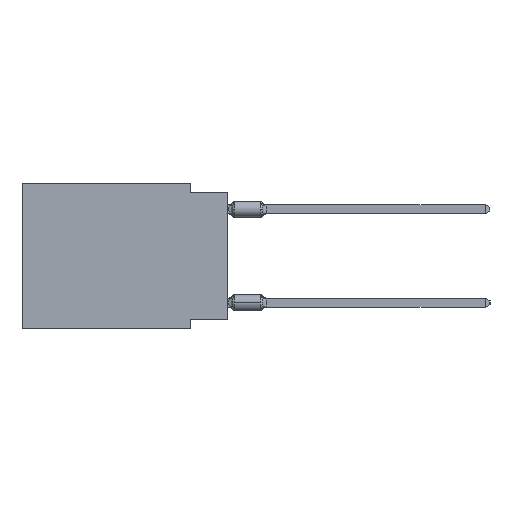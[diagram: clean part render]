
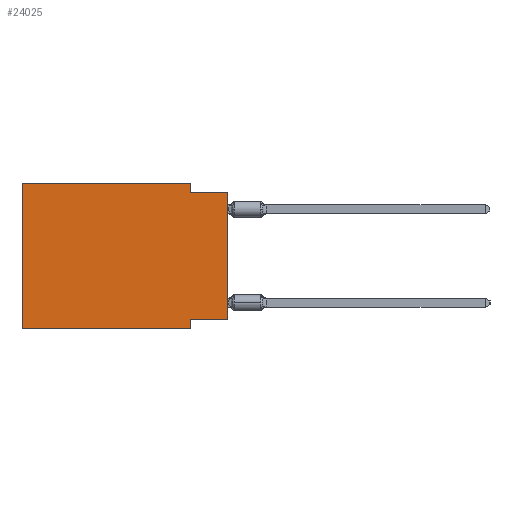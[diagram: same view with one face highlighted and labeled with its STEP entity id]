
A CAD part, left-side view. The second image highlights one B-rep face of the part: STEP entity #24025.
In plain terms, the highlighted planar face has unit normal (-1, 0, 0).
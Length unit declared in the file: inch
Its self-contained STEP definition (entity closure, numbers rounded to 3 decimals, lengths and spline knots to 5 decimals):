
#186 = DIRECTION ( 'NONE',  ( 0., 0., -1. ) ) ;
#632 = LINE ( 'NONE', #25896, #49363 ) ;
#1411 = EDGE_CURVE ( 'NONE', #21787, #33160, #45205, .T. ) ;
#2446 = LINE ( 'NONE', #11648, #55852 ) ;
#2876 = DIRECTION ( 'NONE',  ( 0., -1., 0. ) ) ;
#4531 = EDGE_CURVE ( 'NONE', #33160, #37035, #17638, .T. ) ;
#4639 = VERTEX_POINT ( 'NONE', #9086 ) ;
#4641 = LINE ( 'NONE', #53505, #16126 ) ;
#7725 = VECTOR ( 'NONE', #46171, 39.37008 ) ;
#8576 = VECTOR ( 'NONE', #23397, 39.37008 ) ;
#9086 = CARTESIAN_POINT ( 'NONE',  ( 0., 0.55, -0.39 ) ) ;
#10463 = EDGE_CURVE ( 'NONE', #4639, #32710, #58477, .T. ) ;
#11090 = CARTESIAN_POINT ( 'NONE',  ( 0., 0.1, 0. ) ) ;
#11648 = CARTESIAN_POINT ( 'NONE',  ( 0., 0.55, 0. ) ) ;
#12163 = EDGE_CURVE ( 'NONE', #59722, #14822, #4641, .T. ) ;
#12637 = EDGE_LOOP ( 'NONE', ( #64023, #55850, #13127, #46720, #32402, #53237, #25804, #24884 ) ) ;
#12735 = CARTESIAN_POINT ( 'NONE',  ( 0., 0., -0.025 ) ) ;
#13127 = ORIENTED_EDGE ( 'NONE', *, *, #1411, .F. ) ;
#14822 = VERTEX_POINT ( 'NONE', #28301 ) ;
#16050 = DIRECTION ( 'NONE',  ( 0., -1., 0. ) ) ;
#16126 = VECTOR ( 'NONE', #24639, 39.37008 ) ;
#16457 = CARTESIAN_POINT ( 'NONE',  ( 0., 0.1, -0.025 ) ) ;
#17084 = CARTESIAN_POINT ( 'NONE',  ( 0., 0.1, -0.39 ) ) ;
#17638 = LINE ( 'NONE', #12735, #24336 ) ;
#20513 = PLANE ( 'NONE',  #43126 ) ;
#21787 = VERTEX_POINT ( 'NONE', #56785 ) ;
#23397 = DIRECTION ( 'NONE',  ( 0., 0., 1. ) ) ;
#24025 = ADVANCED_FACE ( 'NONE', ( #35272 ), #20513, .F. ) ;
#24336 = VECTOR ( 'NONE', #2876, 39.37008 ) ;
#24639 = DIRECTION ( 'NONE',  ( 0., 1., 0. ) ) ;
#24884 = ORIENTED_EDGE ( 'NONE', *, *, #12163, .F. ) ;
#25804 = ORIENTED_EDGE ( 'NONE', *, *, #47475, .F. ) ;
#25896 = CARTESIAN_POINT ( 'NONE',  ( 0., 0.55, -0.39 ) ) ;
#27677 = EDGE_CURVE ( 'NONE', #32710, #21787, #2446, .T. ) ;
#28301 = CARTESIAN_POINT ( 'NONE',  ( 0., 0.1, -0.365 ) ) ;
#29759 = VECTOR ( 'NONE', #56361, 39.37008 ) ;
#32402 = ORIENTED_EDGE ( 'NONE', *, *, #10463, .F. ) ;
#32710 = VERTEX_POINT ( 'NONE', #53068 ) ;
#32928 = VECTOR ( 'NONE', #47964, 39.37008 ) ;
#33160 = VERTEX_POINT ( 'NONE', #16457 ) ;
#35272 = FACE_OUTER_BOUND ( 'NONE', #12637, .T. ) ;
#35713 = CARTESIAN_POINT ( 'NONE',  ( 0., 0.1, -0.39 ) ) ;
#37035 = VERTEX_POINT ( 'NONE', #61209 ) ;
#41490 = DIRECTION ( 'NONE',  ( 0., -1., 0. ) ) ;
#42134 = EDGE_CURVE ( 'NONE', #4639, #54829, #632, .T. ) ;
#43126 = AXIS2_PLACEMENT_3D ( 'NONE', #45112, #62066, #186 ) ;
#45112 = CARTESIAN_POINT ( 'NONE',  ( 0., 0.55, 0. ) ) ;
#45205 = LINE ( 'NONE', #11090, #7725 ) ;
#45882 = LINE ( 'NONE', #35713, #29759 ) ;
#46171 = DIRECTION ( 'NONE',  ( 0., 0., -1. ) ) ;
#46720 = ORIENTED_EDGE ( 'NONE', *, *, #27677, .F. ) ;
#47475 = EDGE_CURVE ( 'NONE', #14822, #54829, #45882, .T. ) ;
#47944 = EDGE_CURVE ( 'NONE', #59722, #37035, #48612, .T. ) ;
#47964 = DIRECTION ( 'NONE',  ( 0., 0., 1. ) ) ;
#48612 = LINE ( 'NONE', #48935, #32928 ) ;
#48935 = CARTESIAN_POINT ( 'NONE',  ( 0., 0., 0. ) ) ;
#49293 = CARTESIAN_POINT ( 'NONE',  ( 0., 0.55, 0. ) ) ;
#49363 = VECTOR ( 'NONE', #16050, 39.37008 ) ;
#53068 = CARTESIAN_POINT ( 'NONE',  ( 0., 0.55, 0. ) ) ;
#53237 = ORIENTED_EDGE ( 'NONE', *, *, #42134, .T. ) ;
#53505 = CARTESIAN_POINT ( 'NONE',  ( 0., 0., -0.365 ) ) ;
#54829 = VERTEX_POINT ( 'NONE', #17084 ) ;
#55850 = ORIENTED_EDGE ( 'NONE', *, *, #4531, .F. ) ;
#55852 = VECTOR ( 'NONE', #41490, 39.37008 ) ;
#56361 = DIRECTION ( 'NONE',  ( 0., 0., -1. ) ) ;
#56785 = CARTESIAN_POINT ( 'NONE',  ( 0., 0.1, 0. ) ) ;
#58477 = LINE ( 'NONE', #49293, #8576 ) ;
#59722 = VERTEX_POINT ( 'NONE', #60958 ) ;
#60958 = CARTESIAN_POINT ( 'NONE',  ( 0., 0., -0.365 ) ) ;
#61209 = CARTESIAN_POINT ( 'NONE',  ( 0., 0., -0.025 ) ) ;
#62066 = DIRECTION ( 'NONE',  ( 1., 0., 0. ) ) ;
#64023 = ORIENTED_EDGE ( 'NONE', *, *, #47944, .T. ) ;
